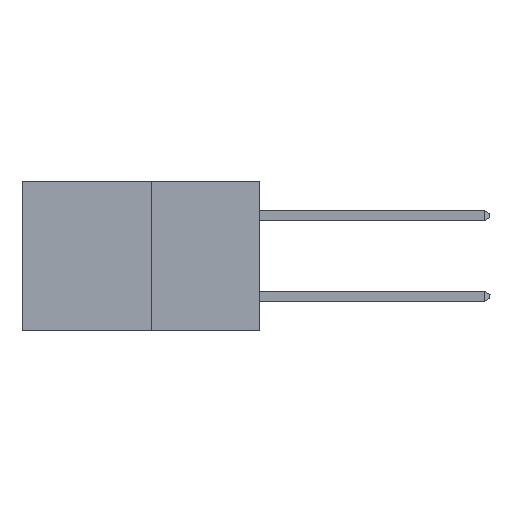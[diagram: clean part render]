
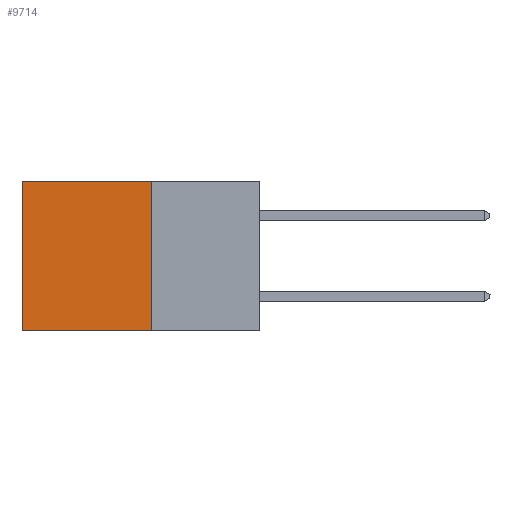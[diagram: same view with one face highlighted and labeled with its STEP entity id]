
A CAD part, left-side view. The second image highlights one B-rep face of the part: STEP entity #9714.
In plain terms, the highlighted planar face has unit normal (-1, 0, 0).
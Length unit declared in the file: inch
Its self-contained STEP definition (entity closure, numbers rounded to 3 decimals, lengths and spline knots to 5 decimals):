
#950 = CARTESIAN_POINT ( 'NONE',  ( 0.277, 0.27, -0.37 ) ) ;
#2564 = EDGE_CURVE ( 'NONE', #6134, #20983, #22495, .T. ) ;
#3009 = CARTESIAN_POINT ( 'NONE',  ( 0.277, 0.59, -0.37 ) ) ;
#3337 = CARTESIAN_POINT ( 'NONE',  ( 0.277, 0.27, -0.37 ) ) ;
#4391 = EDGE_LOOP ( 'NONE', ( #18607, #10496, #22602, #13401 ) ) ;
#4733 = CARTESIAN_POINT ( 'NONE',  ( 0.277, 0.27, -0.37 ) ) ;
#5267 = DIRECTION ( 'NONE',  ( 0., 0., -1. ) ) ;
#5553 = LINE ( 'NONE', #3009, #19783 ) ;
#6134 = VERTEX_POINT ( 'NONE', #950 ) ;
#6219 = VERTEX_POINT ( 'NONE', #20360 ) ;
#6510 = VECTOR ( 'NONE', #10373, 39.37008 ) ;
#6517 = CARTESIAN_POINT ( 'NONE',  ( 0.277, 0.59, -0.37 ) ) ;
#6687 = CARTESIAN_POINT ( 'NONE',  ( 0.277, 0.27, 0. ) ) ;
#7731 = VECTOR ( 'NONE', #8836, 39.37008 ) ;
#8658 = CARTESIAN_POINT ( 'NONE',  ( 0.277, 0.27, -0.37 ) ) ;
#8836 = DIRECTION ( 'NONE',  ( 0., 1., 0. ) ) ;
#9714 = ADVANCED_FACE ( 'NONE', ( #12848 ), #12656, .F. ) ;
#10303 = EDGE_CURVE ( 'NONE', #6219, #20983, #5553, .T. ) ;
#10373 = DIRECTION ( 'NONE',  ( 0., 0., -1. ) ) ;
#10496 = ORIENTED_EDGE ( 'NONE', *, *, #2564, .F. ) ;
#11947 = CARTESIAN_POINT ( 'NONE',  ( 0.277, 0.27, 0. ) ) ;
#12656 = PLANE ( 'NONE',  #12699 ) ;
#12699 = AXIS2_PLACEMENT_3D ( 'NONE', #3337, #16371, #5267 ) ;
#12848 = FACE_OUTER_BOUND ( 'NONE', #4391, .T. ) ;
#13401 = ORIENTED_EDGE ( 'NONE', *, *, #14362, .T. ) ;
#14362 = EDGE_CURVE ( 'NONE', #15997, #6219, #17332, .T. ) ;
#15997 = VERTEX_POINT ( 'NONE', #11947 ) ;
#16024 = DIRECTION ( 'NONE',  ( 0., 0., -1. ) ) ;
#16371 = DIRECTION ( 'NONE',  ( 1., 0., 0. ) ) ;
#17332 = LINE ( 'NONE', #6687, #21649 ) ;
#18607 = ORIENTED_EDGE ( 'NONE', *, *, #10303, .T. ) ;
#19027 = EDGE_CURVE ( 'NONE', #15997, #6134, #21308, .T. ) ;
#19783 = VECTOR ( 'NONE', #16024, 39.37008 ) ;
#20360 = CARTESIAN_POINT ( 'NONE',  ( 0.277, 0.59, 0. ) ) ;
#20983 = VERTEX_POINT ( 'NONE', #6517 ) ;
#21308 = LINE ( 'NONE', #4733, #6510 ) ;
#21649 = VECTOR ( 'NONE', #23319, 39.37008 ) ;
#22495 = LINE ( 'NONE', #8658, #7731 ) ;
#22602 = ORIENTED_EDGE ( 'NONE', *, *, #19027, .F. ) ;
#23319 = DIRECTION ( 'NONE',  ( 0., 1., 0. ) ) ;
